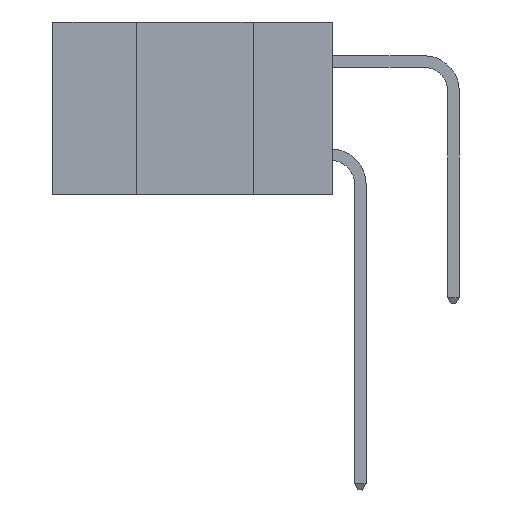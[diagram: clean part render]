
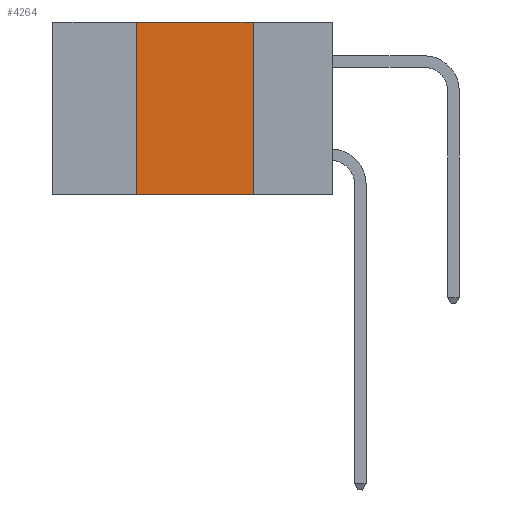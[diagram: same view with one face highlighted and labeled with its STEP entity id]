
A CAD part, left-side view. The second image highlights one B-rep face of the part: STEP entity #4264.
In plain terms, the highlighted planar face has unit normal (-1, 0, 0).
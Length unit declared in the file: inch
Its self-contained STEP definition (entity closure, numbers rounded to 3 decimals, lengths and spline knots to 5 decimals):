
#2121 = VECTOR ( 'NONE', #15188, 39.37008 ) ;
#2386 = CARTESIAN_POINT ( 'NONE',  ( 0., 0.17, 0. ) ) ;
#2559 = FACE_OUTER_BOUND ( 'NONE', #19258, .T. ) ;
#2995 = EDGE_CURVE ( 'NONE', #4711, #8813, #14642, .T. ) ;
#3064 = CARTESIAN_POINT ( 'NONE',  ( 0., 0.6, -0.37 ) ) ;
#4162 = CARTESIAN_POINT ( 'NONE',  ( 0., 0.17, 0. ) ) ;
#4264 = ADVANCED_FACE ( 'NONE', ( #2559 ), #15349, .F. ) ;
#4711 = VERTEX_POINT ( 'NONE', #9178 ) ;
#4758 = CARTESIAN_POINT ( 'NONE',  ( 0., 0.42, 0. ) ) ;
#5225 = VERTEX_POINT ( 'NONE', #2386 ) ;
#5649 = VECTOR ( 'NONE', #9295, 39.37008 ) ;
#5732 = DIRECTION ( 'NONE',  ( 0., 0., -1. ) ) ;
#5783 = LINE ( 'NONE', #8385, #8928 ) ;
#8385 = CARTESIAN_POINT ( 'NONE',  ( 0., 0.6, 0. ) ) ;
#8813 = VERTEX_POINT ( 'NONE', #4758 ) ;
#8928 = VECTOR ( 'NONE', #16155, 39.37008 ) ;
#9178 = CARTESIAN_POINT ( 'NONE',  ( 0., 0.42, -0.37 ) ) ;
#9295 = DIRECTION ( 'NONE',  ( 0., -1., 0. ) ) ;
#9741 = LINE ( 'NONE', #3064, #5649 ) ;
#10114 = VECTOR ( 'NONE', #5732, 39.37008 ) ;
#11765 = CARTESIAN_POINT ( 'NONE',  ( 0., 0.17, -0.37 ) ) ;
#12988 = ORIENTED_EDGE ( 'NONE', *, *, #2995, .F. ) ;
#13196 = ORIENTED_EDGE ( 'NONE', *, *, #19231, .T. ) ;
#13729 = ORIENTED_EDGE ( 'NONE', *, *, #15814, .F. ) ;
#14642 = LINE ( 'NONE', #17590, #2121 ) ;
#15083 = ORIENTED_EDGE ( 'NONE', *, *, #15317, .F. ) ;
#15188 = DIRECTION ( 'NONE',  ( 0., 0., 1. ) ) ;
#15317 = EDGE_CURVE ( 'NONE', #5225, #15936, #18328, .T. ) ;
#15349 = PLANE ( 'NONE',  #18134 ) ;
#15814 = EDGE_CURVE ( 'NONE', #8813, #5225, #5783, .T. ) ;
#15936 = VERTEX_POINT ( 'NONE', #11765 ) ;
#16155 = DIRECTION ( 'NONE',  ( 0., -1., 0. ) ) ;
#16318 = DIRECTION ( 'NONE',  ( 0., 0., -1. ) ) ;
#16400 = DIRECTION ( 'NONE',  ( 1., 0., 0. ) ) ;
#17590 = CARTESIAN_POINT ( 'NONE',  ( 0., 0.42, 0. ) ) ;
#18134 = AXIS2_PLACEMENT_3D ( 'NONE', #20162, #16400, #16318 ) ;
#18328 = LINE ( 'NONE', #4162, #10114 ) ;
#19231 = EDGE_CURVE ( 'NONE', #4711, #15936, #9741, .T. ) ;
#19258 = EDGE_LOOP ( 'NONE', ( #15083, #13729, #12988, #13196 ) ) ;
#20162 = CARTESIAN_POINT ( 'NONE',  ( 0., 0.6, 0. ) ) ;
